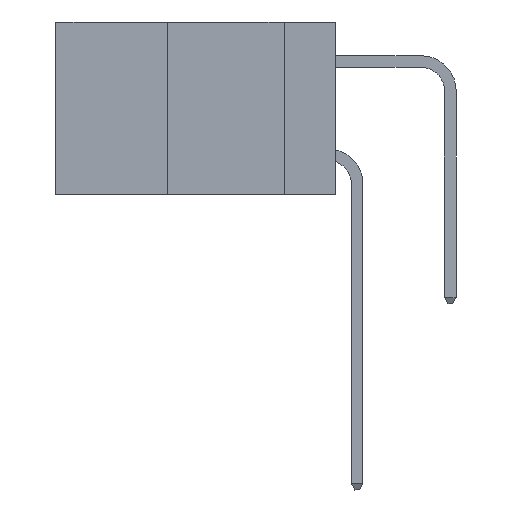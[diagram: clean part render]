
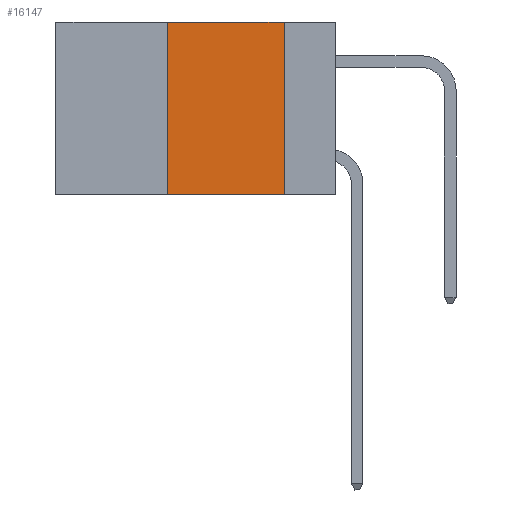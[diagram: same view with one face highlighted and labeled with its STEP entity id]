
A CAD part, left-side view. The second image highlights one B-rep face of the part: STEP entity #16147.
In plain terms, the highlighted planar face has unit normal (-1, 0, 0).
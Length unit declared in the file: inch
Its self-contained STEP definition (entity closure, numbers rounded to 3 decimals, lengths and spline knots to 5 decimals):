
#6 = ORIENTED_EDGE ( 'NONE', *, *, #20596, .F. ) ;
#936 = EDGE_CURVE ( 'NONE', #18175, #13494, #6813, .T. ) ;
#1181 = VERTEX_POINT ( 'NONE', #10694 ) ;
#1951 = VECTOR ( 'NONE', #10654, 39.37008 ) ;
#3129 = EDGE_CURVE ( 'NONE', #18175, #11061, #22039, .T. ) ;
#3229 = CARTESIAN_POINT ( 'NONE',  ( 0., 0.11, -0.37 ) ) ;
#3551 = PLANE ( 'NONE',  #11233 ) ;
#4924 = CARTESIAN_POINT ( 'NONE',  ( 0., 0.11, 0. ) ) ;
#5047 = DIRECTION ( 'NONE',  ( 1., 0., 0. ) ) ;
#5163 = DIRECTION ( 'NONE',  ( 0., 0., -1. ) ) ;
#5853 = CARTESIAN_POINT ( 'NONE',  ( 0., 0.36, 0. ) ) ;
#6719 = CARTESIAN_POINT ( 'NONE',  ( 0., 0.36, -0.37 ) ) ;
#6813 = LINE ( 'NONE', #19493, #13771 ) ;
#8624 = DIRECTION ( 'NONE',  ( 0., -1., 0. ) ) ;
#9419 = LINE ( 'NONE', #14809, #21284 ) ;
#10013 = ORIENTED_EDGE ( 'NONE', *, *, #936, .T. ) ;
#10654 = DIRECTION ( 'NONE',  ( 0., 0., -1. ) ) ;
#10694 = CARTESIAN_POINT ( 'NONE',  ( 0., 0.11, 0. ) ) ;
#11061 = VERTEX_POINT ( 'NONE', #5853 ) ;
#11233 = AXIS2_PLACEMENT_3D ( 'NONE', #16275, #5047, #5163 ) ;
#11955 = CARTESIAN_POINT ( 'NONE',  ( 0., 0.36, 0. ) ) ;
#12168 = VECTOR ( 'NONE', #15757, 39.37008 ) ;
#12727 = LINE ( 'NONE', #4924, #1951 ) ;
#13225 = EDGE_LOOP ( 'NONE', ( #6, #14044, #14445, #10013 ) ) ;
#13494 = VERTEX_POINT ( 'NONE', #3229 ) ;
#13696 = EDGE_CURVE ( 'NONE', #11061, #1181, #9419, .T. ) ;
#13771 = VECTOR ( 'NONE', #8624, 39.37008 ) ;
#14044 = ORIENTED_EDGE ( 'NONE', *, *, #13696, .F. ) ;
#14445 = ORIENTED_EDGE ( 'NONE', *, *, #3129, .F. ) ;
#14809 = CARTESIAN_POINT ( 'NONE',  ( 0., 0.6, 0. ) ) ;
#15757 = DIRECTION ( 'NONE',  ( 0., 0., 1. ) ) ;
#16147 = ADVANCED_FACE ( 'NONE', ( #16384 ), #3551, .F. ) ;
#16275 = CARTESIAN_POINT ( 'NONE',  ( 0., 0.6, 0. ) ) ;
#16384 = FACE_OUTER_BOUND ( 'NONE', #13225, .T. ) ;
#16862 = DIRECTION ( 'NONE',  ( 0., -1., 0. ) ) ;
#18175 = VERTEX_POINT ( 'NONE', #6719 ) ;
#19493 = CARTESIAN_POINT ( 'NONE',  ( 0., 0.6, -0.37 ) ) ;
#20596 = EDGE_CURVE ( 'NONE', #1181, #13494, #12727, .T. ) ;
#21284 = VECTOR ( 'NONE', #16862, 39.37008 ) ;
#22039 = LINE ( 'NONE', #11955, #12168 ) ;
